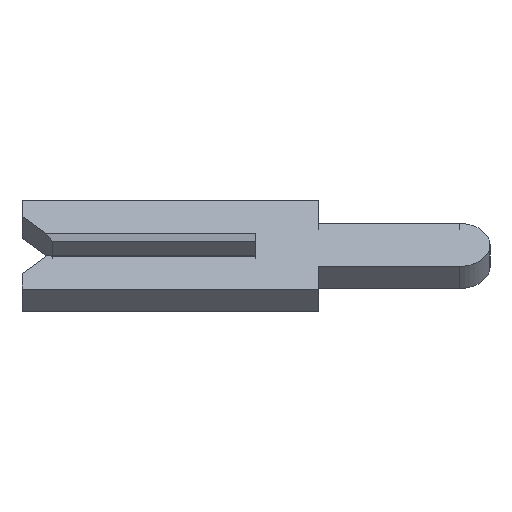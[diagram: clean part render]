
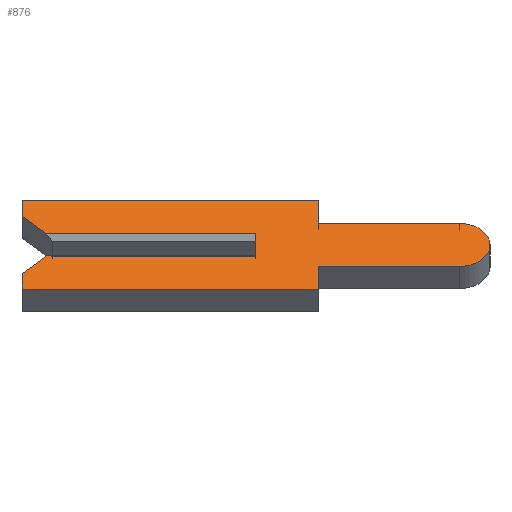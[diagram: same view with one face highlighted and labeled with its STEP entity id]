
A CAD part, left-side view. The second image highlights one B-rep face of the part: STEP entity #876.
In plain terms, the highlighted face is planar.
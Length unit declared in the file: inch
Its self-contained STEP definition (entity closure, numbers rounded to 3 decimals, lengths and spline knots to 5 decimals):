
#15 = CARTESIAN_POINT ( 'NONE',  ( -0.01, 0., -0.01 ) ) ;
#26 = ORIENTED_EDGE ( 'NONE', *, *, #664, .F. ) ;
#49 = EDGE_CURVE ( 'NONE', #382, #697, #1123, .T. ) ;
#62 = VERTEX_POINT ( 'NONE', #1363 ) ;
#102 = VERTEX_POINT ( 'NONE', #210 ) ;
#106 = DIRECTION ( 'NONE',  ( 0., 0., 1. ) ) ;
#118 = CARTESIAN_POINT ( 'NONE',  ( -0.01, -0.1305, 0.0195 ) ) ;
#123 = VERTEX_POINT ( 'NONE', #118 ) ;
#137 = AXIS2_PLACEMENT_3D ( 'NONE', #946, #810, #148 ) ;
#138 = ORIENTED_EDGE ( 'NONE', *, *, #584, .F. ) ;
#148 = DIRECTION ( 'NONE',  ( 0., 0., -1. ) ) ;
#162 = LINE ( 'NONE', #846, #991 ) ;
#169 = VECTOR ( 'NONE', #985, 39.37008 ) ;
#171 = PLANE ( 'NONE',  #480 ) ;
#177 = LINE ( 'NONE', #1122, #974 ) ;
#180 = LINE ( 'NONE', #914, #1015 ) ;
#186 = CARTESIAN_POINT ( 'NONE',  ( -0.01, 0., 0.01 ) ) ;
#194 = ORIENTED_EDGE ( 'NONE', *, *, #598, .F. ) ;
#207 = ORIENTED_EDGE ( 'NONE', *, *, #1233, .F. ) ;
#210 = CARTESIAN_POINT ( 'NONE',  ( -0.01, 0.15, 0.026 ) ) ;
#239 = CARTESIAN_POINT ( 'NONE',  ( -0.01, 0.134, 0.01 ) ) ;
#247 = VECTOR ( 'NONE', #942, 39.37008 ) ;
#253 = DIRECTION ( 'NONE',  ( 0., 0.707, 0.707 ) ) ;
#286 = ORIENTED_EDGE ( 'NONE', *, *, #1035, .F. ) ;
#289 = CARTESIAN_POINT ( 'NONE',  ( -0.01, -0.1305, -0.01 ) ) ;
#296 = LINE ( 'NONE', #1279, #247 ) ;
#315 = ORIENTED_EDGE ( 'NONE', *, *, #1397, .F. ) ;
#317 = CIRCLE ( 'NONE', #137, 0.0195 ) ;
#320 = EDGE_LOOP ( 'NONE', ( #530, #444, #833, #315, #1011, #138, #207, #286, #194, #26, #422, #333, #352, #1049 ) ) ;
#333 = ORIENTED_EDGE ( 'NONE', *, *, #943, .F. ) ;
#352 = ORIENTED_EDGE ( 'NONE', *, *, #1388, .F. ) ;
#374 = EDGE_CURVE ( 'NONE', #1406, #1298, #180, .T. ) ;
#382 = VERTEX_POINT ( 'NONE', #15 ) ;
#395 = CARTESIAN_POINT ( 'NONE',  ( -0.01, -0.04, -0.04 ) ) ;
#409 = DIRECTION ( 'NONE',  ( 0., 0., -1. ) ) ;
#413 = CARTESIAN_POINT ( 'NONE',  ( -0.01, -0.04, -0.04 ) ) ;
#422 = ORIENTED_EDGE ( 'NONE', *, *, #374, .F. ) ;
#444 = ORIENTED_EDGE ( 'NONE', *, *, #49, .F. ) ;
#461 = EDGE_CURVE ( 'NONE', #1356, #102, #535, .T. ) ;
#480 = AXIS2_PLACEMENT_3D ( 'NONE', #1306, #1062, #409 ) ;
#493 = DIRECTION ( 'NONE',  ( 0., 1., 0. ) ) ;
#512 = DIRECTION ( 'NONE',  ( 0., -1., 0. ) ) ;
#515 = VECTOR ( 'NONE', #1235, 39.37008 ) ;
#530 = ORIENTED_EDGE ( 'NONE', *, *, #1068, .T. ) ;
#534 = CARTESIAN_POINT ( 'NONE',  ( -0.01, -0.04, -0.0195 ) ) ;
#535 = LINE ( 'NONE', #785, #783 ) ;
#537 = FACE_OUTER_BOUND ( 'NONE', #320, .T. ) ;
#539 = CARTESIAN_POINT ( 'NONE',  ( -0.01, 0.15, -0.026 ) ) ;
#547 = DIRECTION ( 'NONE',  ( 0., -0.707, 0.707 ) ) ;
#584 = EDGE_CURVE ( 'NONE', #958, #747, #1282, .T. ) ;
#598 = EDGE_CURVE ( 'NONE', #123, #797, #317, .T. ) ;
#604 = EDGE_CURVE ( 'NONE', #747, #1030, #635, .T. ) ;
#606 = VECTOR ( 'NONE', #547, 39.37008 ) ;
#635 = LINE ( 'NONE', #930, #1210 ) ;
#661 = LINE ( 'NONE', #289, #1289 ) ;
#664 = EDGE_CURVE ( 'NONE', #1298, #123, #296, .T. ) ;
#675 = CARTESIAN_POINT ( 'NONE',  ( -0.01, -0.04, 0.04 ) ) ;
#694 = VECTOR ( 'NONE', #493, 39.37008 ) ;
#697 = VERTEX_POINT ( 'NONE', #186 ) ;
#724 = DIRECTION ( 'NONE',  ( 0., -1., 0. ) ) ;
#738 = CARTESIAN_POINT ( 'NONE',  ( -0.01, -0.1305, -0.0195 ) ) ;
#747 = VERTEX_POINT ( 'NONE', #1073 ) ;
#750 = EDGE_CURVE ( 'NONE', #62, #382, #661, .T. ) ;
#752 = VECTOR ( 'NONE', #1103, 39.37008 ) ;
#768 = CARTESIAN_POINT ( 'NONE',  ( -0.01, 0.1305, -0.0065 ) ) ;
#783 = VECTOR ( 'NONE', #253, 39.37008 ) ;
#785 = CARTESIAN_POINT ( 'NONE',  ( -0.01, 0.1305, 0.0065 ) ) ;
#797 = VERTEX_POINT ( 'NONE', #738 ) ;
#809 = VECTOR ( 'NONE', #859, 39.37008 ) ;
#810 = DIRECTION ( 'NONE',  ( 1., 0., 0. ) ) ;
#833 = ORIENTED_EDGE ( 'NONE', *, *, #750, .F. ) ;
#846 = CARTESIAN_POINT ( 'NONE',  ( -0.01, 0.15, 0.04 ) ) ;
#859 = DIRECTION ( 'NONE',  ( 0., 1., 0. ) ) ;
#874 = CARTESIAN_POINT ( 'NONE',  ( -0.01, 0.15, 0.01 ) ) ;
#876 = ADVANCED_FACE ( 'NONE', ( #537 ), #171, .F. ) ;
#914 = CARTESIAN_POINT ( 'NONE',  ( -0.01, -0.04, 0.04 ) ) ;
#924 = DIRECTION ( 'NONE',  ( 0., 0., 1. ) ) ;
#930 = CARTESIAN_POINT ( 'NONE',  ( -0.01, 0.15, -0.026 ) ) ;
#942 = DIRECTION ( 'NONE',  ( 0., -1., 0. ) ) ;
#943 = EDGE_CURVE ( 'NONE', #956, #1406, #162, .T. ) ;
#946 = CARTESIAN_POINT ( 'NONE',  ( -0.01, -0.1305, 0. ) ) ;
#956 = VERTEX_POINT ( 'NONE', #1410 ) ;
#958 = VERTEX_POINT ( 'NONE', #395 ) ;
#973 = CARTESIAN_POINT ( 'NONE',  ( -0.01, -0.04, -0.0195 ) ) ;
#974 = VECTOR ( 'NONE', #106, 39.37008 ) ;
#985 = DIRECTION ( 'NONE',  ( 0., -1., 0. ) ) ;
#991 = VECTOR ( 'NONE', #724, 39.37008 ) ;
#1008 = CARTESIAN_POINT ( 'NONE',  ( -0.01, 0., 0.0065 ) ) ;
#1011 = ORIENTED_EDGE ( 'NONE', *, *, #604, .F. ) ;
#1015 = VECTOR ( 'NONE', #1145, 39.37008 ) ;
#1030 = VERTEX_POINT ( 'NONE', #539 ) ;
#1035 = EDGE_CURVE ( 'NONE', #797, #1140, #1115, .T. ) ;
#1049 = ORIENTED_EDGE ( 'NONE', *, *, #461, .F. ) ;
#1062 = DIRECTION ( 'NONE',  ( 1., 0., 0. ) ) ;
#1068 = EDGE_CURVE ( 'NONE', #1356, #697, #1095, .T. ) ;
#1073 = CARTESIAN_POINT ( 'NONE',  ( -0.01, 0.15, -0.04 ) ) ;
#1095 = LINE ( 'NONE', #874, #169 ) ;
#1103 = DIRECTION ( 'NONE',  ( 0., 0., -1. ) ) ;
#1115 = LINE ( 'NONE', #534, #809 ) ;
#1122 = CARTESIAN_POINT ( 'NONE',  ( -0.01, 0.15, 0.026 ) ) ;
#1123 = LINE ( 'NONE', #1008, #515 ) ;
#1140 = VERTEX_POINT ( 'NONE', #973 ) ;
#1145 = DIRECTION ( 'NONE',  ( 0., 0., -1. ) ) ;
#1174 = CARTESIAN_POINT ( 'NONE',  ( -0.01, 0.15, -0.04 ) ) ;
#1195 = LINE ( 'NONE', #768, #606 ) ;
#1210 = VECTOR ( 'NONE', #924, 39.37008 ) ;
#1233 = EDGE_CURVE ( 'NONE', #1140, #958, #1368, .T. ) ;
#1235 = DIRECTION ( 'NONE',  ( 0., 0., 1. ) ) ;
#1279 = CARTESIAN_POINT ( 'NONE',  ( -0.01, -0.04, 0.0195 ) ) ;
#1282 = LINE ( 'NONE', #1174, #694 ) ;
#1289 = VECTOR ( 'NONE', #512, 39.37008 ) ;
#1298 = VERTEX_POINT ( 'NONE', #1319 ) ;
#1306 = CARTESIAN_POINT ( 'NONE',  ( -0.01, -0.1305, 0. ) ) ;
#1319 = CARTESIAN_POINT ( 'NONE',  ( -0.01, -0.04, 0.0195 ) ) ;
#1356 = VERTEX_POINT ( 'NONE', #239 ) ;
#1363 = CARTESIAN_POINT ( 'NONE',  ( -0.01, 0.134, -0.01 ) ) ;
#1368 = LINE ( 'NONE', #413, #752 ) ;
#1388 = EDGE_CURVE ( 'NONE', #102, #956, #177, .T. ) ;
#1397 = EDGE_CURVE ( 'NONE', #1030, #62, #1195, .T. ) ;
#1406 = VERTEX_POINT ( 'NONE', #675 ) ;
#1410 = CARTESIAN_POINT ( 'NONE',  ( -0.01, 0.15, 0.04 ) ) ;
